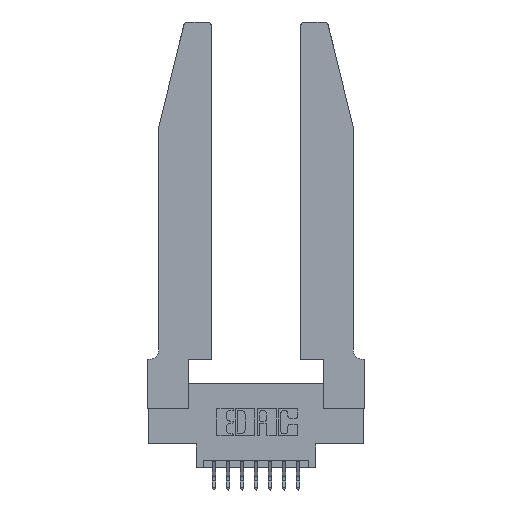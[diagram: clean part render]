
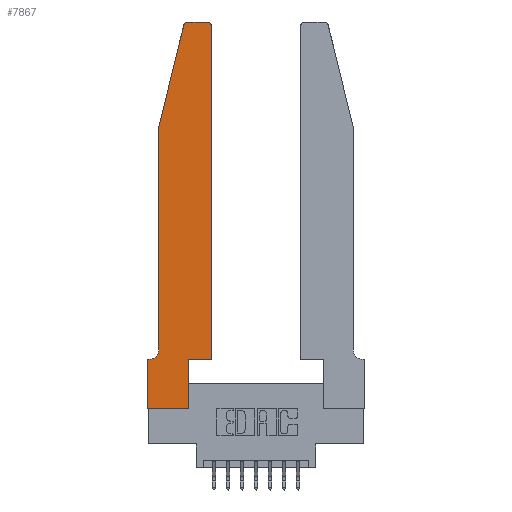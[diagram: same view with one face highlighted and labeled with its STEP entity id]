
A CAD part, top view. The second image highlights one B-rep face of the part: STEP entity #7867.
In plain terms, the highlighted planar face has unit normal (0, 0, 1).
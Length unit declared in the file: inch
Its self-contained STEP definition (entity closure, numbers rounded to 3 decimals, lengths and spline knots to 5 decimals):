
#195 = EDGE_CURVE ( 'NONE', #11717, #13821, #14952, .T. ) ;
#417 = LINE ( 'NONE', #14870, #12669 ) ;
#590 = CARTESIAN_POINT ( 'NONE',  ( 0.4505, 0.35, 0.37 ) ) ;
#743 = DIRECTION ( 'NONE',  ( 0., 1., 0. ) ) ;
#755 = DIRECTION ( 'NONE',  ( -0.239, -0.971, 0. ) ) ;
#758 = LINE ( 'NONE', #13718, #13002 ) ;
#879 = CARTESIAN_POINT ( 'NONE',  ( 0.4505, 2.72, 0.37 ) ) ;
#1035 = EDGE_CURVE ( 'NONE', #8137, #13142, #1864, .T. ) ;
#1266 = CIRCLE ( 'NONE', #7705, 0.03 ) ;
#1410 = EDGE_CURVE ( 'NONE', #7288, #7017, #758, .T. ) ;
#1479 = ORIENTED_EDGE ( 'NONE', *, *, #1035, .T. ) ;
#1484 = VECTOR ( 'NONE', #2239, 39.37008 ) ;
#1756 = ORIENTED_EDGE ( 'NONE', *, *, #5310, .T. ) ;
#1829 = VECTOR ( 'NONE', #9307, 39.37008 ) ;
#1864 = LINE ( 'NONE', #8002, #1484 ) ;
#2239 = DIRECTION ( 'NONE',  ( 1., 0., 0. ) ) ;
#2380 = CARTESIAN_POINT ( 'NONE',  ( 0.0755, 2., 0.37 ) ) ;
#3016 = VERTEX_POINT ( 'NONE', #7298 ) ;
#3124 = CARTESIAN_POINT ( 'NONE',  ( 0.4205, 2.72, 0.37 ) ) ;
#3308 = EDGE_LOOP ( 'NONE', ( #12075, #9357, #14810, #13504, #5225, #4441, #1756, #1479, #6377, #12096, #7942, #7580 ) ) ;
#3467 = DIRECTION ( 'NONE',  ( -1., 0., 0. ) ) ;
#4093 = VECTOR ( 'NONE', #4187, 39.37008 ) ;
#4187 = DIRECTION ( 'NONE',  ( -1., 0., 0. ) ) ;
#4392 = DIRECTION ( 'NONE',  ( 1., 0., 0. ) ) ;
#4441 = ORIENTED_EDGE ( 'NONE', *, *, #9057, .T. ) ;
#4471 = LINE ( 'NONE', #6576, #4093 ) ;
#4742 = VECTOR ( 'NONE', #3467, 39.37008 ) ;
#4882 = EDGE_CURVE ( 'NONE', #13142, #5454, #417, .T. ) ;
#5225 = ORIENTED_EDGE ( 'NONE', *, *, #195, .T. ) ;
#5288 = EDGE_CURVE ( 'NONE', #3016, #13857, #4471, .T. ) ;
#5310 = EDGE_CURVE ( 'NONE', #8376, #8137, #10307, .T. ) ;
#5358 = EDGE_CURVE ( 'NONE', #10693, #7415, #9234, .T. ) ;
#5454 = VERTEX_POINT ( 'NONE', #12589 ) ;
#5687 = CARTESIAN_POINT ( 'NONE',  ( 0., 0.35, 0.37 ) ) ;
#5720 = FACE_OUTER_BOUND ( 'NONE', #3308, .T. ) ;
#6131 = VECTOR ( 'NONE', #9028, 39.37008 ) ;
#6377 = ORIENTED_EDGE ( 'NONE', *, *, #4882, .T. ) ;
#6431 = CARTESIAN_POINT ( 'NONE',  ( 0.284, 2.72, 0.37 ) ) ;
#6560 = CARTESIAN_POINT ( 'NONE',  ( 0.25487, 2.72718, 0.37 ) ) ;
#6576 = CARTESIAN_POINT ( 'NONE',  ( 0.2605, 2.75, 0.37 ) ) ;
#6871 = DIRECTION ( 'NONE',  ( 1., 0., 0. ) ) ;
#6948 = AXIS2_PLACEMENT_3D ( 'NONE', #6431, #14509, #7647 ) ;
#7017 = VERTEX_POINT ( 'NONE', #13008 ) ;
#7288 = VERTEX_POINT ( 'NONE', #6560 ) ;
#7298 = CARTESIAN_POINT ( 'NONE',  ( 0.4205, 2.75, 0.37 ) ) ;
#7415 = VERTEX_POINT ( 'NONE', #879 ) ;
#7580 = ORIENTED_EDGE ( 'NONE', *, *, #8866, .T. ) ;
#7602 = CARTESIAN_POINT ( 'NONE',  ( 0., 0., 0.37 ) ) ;
#7647 = DIRECTION ( 'NONE',  ( 1., 0., 0. ) ) ;
#7705 = AXIS2_PLACEMENT_3D ( 'NONE', #3124, #11360, #4392 ) ;
#7867 = ADVANCED_FACE ( 'NONE', ( #5720 ), #8011, .T. ) ;
#7893 = LINE ( 'NONE', #10503, #4742 ) ;
#7942 = ORIENTED_EDGE ( 'NONE', *, *, #5358, .T. ) ;
#8002 = CARTESIAN_POINT ( 'NONE',  ( 0., 0., 0.37 ) ) ;
#8011 = PLANE ( 'NONE',  #15029 ) ;
#8137 = VERTEX_POINT ( 'NONE', #7602 ) ;
#8376 = VERTEX_POINT ( 'NONE', #9121 ) ;
#8724 = CARTESIAN_POINT ( 'NONE',  ( 0.0755, 0.42, 0.37 ) ) ;
#8866 = EDGE_CURVE ( 'NONE', #7415, #3016, #1266, .T. ) ;
#8931 = CARTESIAN_POINT ( 'NONE',  ( 0., 0., 0.37 ) ) ;
#9028 = DIRECTION ( 'NONE',  ( 0., 1., 0. ) ) ;
#9035 = EDGE_CURVE ( 'NONE', #5454, #10693, #14350, .T. ) ;
#9057 = EDGE_CURVE ( 'NONE', #13821, #8376, #7893, .T. ) ;
#9121 = CARTESIAN_POINT ( 'NONE',  ( 0., 0.35, 0.37 ) ) ;
#9234 = LINE ( 'NONE', #13592, #6131 ) ;
#9307 = DIRECTION ( 'NONE',  ( 1., 0., 0. ) ) ;
#9357 = ORIENTED_EDGE ( 'NONE', *, *, #12927, .T. ) ;
#9570 = CARTESIAN_POINT ( 'NONE',  ( 0.284, 2.75, 0.37 ) ) ;
#9961 = DIRECTION ( 'NONE',  ( -1., 0., 0. ) ) ;
#10307 = LINE ( 'NONE', #8931, #13031 ) ;
#10460 = CARTESIAN_POINT ( 'NONE',  ( 0.4505, 0.35, 0.37 ) ) ;
#10503 = CARTESIAN_POINT ( 'NONE',  ( 0.0755, 0.35, 0.37 ) ) ;
#10693 = VERTEX_POINT ( 'NONE', #590 ) ;
#11177 = DIRECTION ( 'NONE',  ( 0., 0., -1. ) ) ;
#11213 = DIRECTION ( 'NONE',  ( 0., -1., 0. ) ) ;
#11360 = DIRECTION ( 'NONE',  ( 0., 0., 1. ) ) ;
#11424 = CIRCLE ( 'NONE', #6948, 0.03 ) ;
#11717 = VERTEX_POINT ( 'NONE', #8724 ) ;
#11810 = DIRECTION ( 'NONE',  ( 0., -1., 0. ) ) ;
#12075 = ORIENTED_EDGE ( 'NONE', *, *, #5288, .T. ) ;
#12096 = ORIENTED_EDGE ( 'NONE', *, *, #9035, .T. ) ;
#12589 = CARTESIAN_POINT ( 'NONE',  ( 0.2865, 0.35, 0.37 ) ) ;
#12590 = CARTESIAN_POINT ( 'NONE',  ( 0.2865, 0., 0.37 ) ) ;
#12669 = VECTOR ( 'NONE', #743, 39.37008 ) ;
#12927 = EDGE_CURVE ( 'NONE', #13857, #7288, #11424, .T. ) ;
#13002 = VECTOR ( 'NONE', #755, 39.37008 ) ;
#13008 = CARTESIAN_POINT ( 'NONE',  ( 0.0755, 2., 0.37 ) ) ;
#13031 = VECTOR ( 'NONE', #11213, 39.37008 ) ;
#13142 = VERTEX_POINT ( 'NONE', #12590 ) ;
#13504 = ORIENTED_EDGE ( 'NONE', *, *, #15051, .T. ) ;
#13526 = VECTOR ( 'NONE', #11810, 39.37008 ) ;
#13592 = CARTESIAN_POINT ( 'NONE',  ( 0.4505, 0.35, 0.37 ) ) ;
#13690 = AXIS2_PLACEMENT_3D ( 'NONE', #14285, #11177, #9961 ) ;
#13718 = CARTESIAN_POINT ( 'NONE',  ( 0.0755, 2., 0.37 ) ) ;
#13761 = DIRECTION ( 'NONE',  ( 0., 0., 1. ) ) ;
#13821 = VERTEX_POINT ( 'NONE', #14038 ) ;
#13857 = VERTEX_POINT ( 'NONE', #9570 ) ;
#13894 = LINE ( 'NONE', #2380, #13526 ) ;
#14038 = CARTESIAN_POINT ( 'NONE',  ( 0.0055, 0.35, 0.37 ) ) ;
#14285 = CARTESIAN_POINT ( 'NONE',  ( 0.0055, 0.42, 0.37 ) ) ;
#14350 = LINE ( 'NONE', #10460, #1829 ) ;
#14509 = DIRECTION ( 'NONE',  ( 0., 0., 1. ) ) ;
#14810 = ORIENTED_EDGE ( 'NONE', *, *, #1410, .T. ) ;
#14870 = CARTESIAN_POINT ( 'NONE',  ( 0.2865, 0.35, 0.37 ) ) ;
#14952 = CIRCLE ( 'NONE', #13690, 0.07 ) ;
#15029 = AXIS2_PLACEMENT_3D ( 'NONE', #5687, #13761, #6871 ) ;
#15051 = EDGE_CURVE ( 'NONE', #7017, #11717, #13894, .T. ) ;
